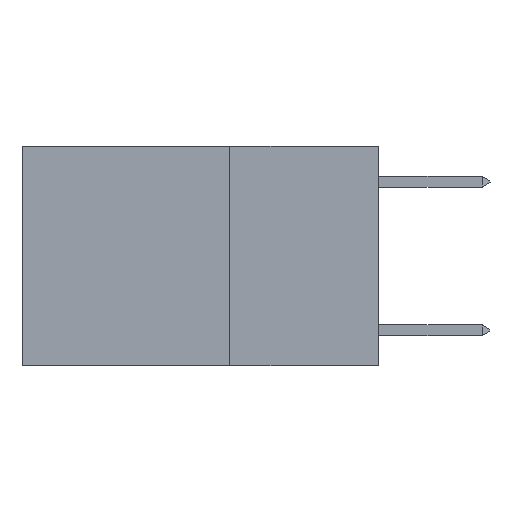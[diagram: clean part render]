
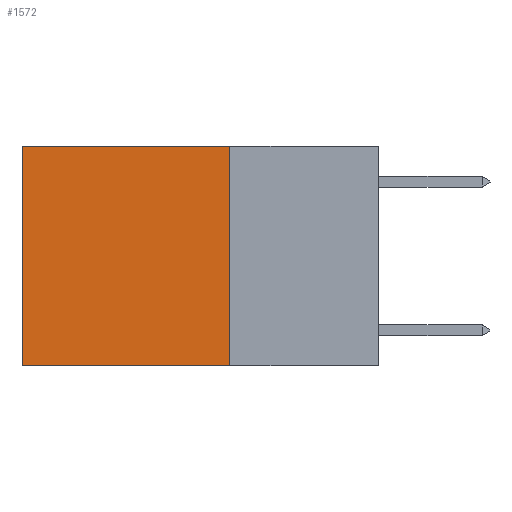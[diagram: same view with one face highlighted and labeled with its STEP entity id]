
A CAD part, left-side view. The second image highlights one B-rep face of the part: STEP entity #1572.
In plain terms, the highlighted planar face has unit normal (-1, 0, 0).
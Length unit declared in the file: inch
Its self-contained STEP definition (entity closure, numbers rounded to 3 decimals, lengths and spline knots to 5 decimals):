
#103 = VECTOR ( 'NONE', #2757, 39.37008 ) ;
#230 = CARTESIAN_POINT ( 'NONE',  ( 0.2625, 0.25, -0.37 ) ) ;
#568 = ORIENTED_EDGE ( 'NONE', *, *, #9293, .T. ) ;
#684 = ORIENTED_EDGE ( 'NONE', *, *, #6577, .F. ) ;
#697 = ORIENTED_EDGE ( 'NONE', *, *, #6767, .F. ) ;
#999 = DIRECTION ( 'NONE',  ( 0., 1., 0. ) ) ;
#1058 = ORIENTED_EDGE ( 'NONE', *, *, #4035, .T. ) ;
#1310 = CARTESIAN_POINT ( 'NONE',  ( 0.2625, 0.6, -0.37 ) ) ;
#1572 = ADVANCED_FACE ( 'NONE', ( #8146 ), #7570, .F. ) ;
#2045 = VECTOR ( 'NONE', #8404, 39.37008 ) ;
#2367 = LINE ( 'NONE', #3501, #2045 ) ;
#2757 = DIRECTION ( 'NONE',  ( 0., 1., 0. ) ) ;
#3449 = LINE ( 'NONE', #6725, #5382 ) ;
#3451 = DIRECTION ( 'NONE',  ( 0., 0., -1. ) ) ;
#3501 = CARTESIAN_POINT ( 'NONE',  ( 0.2625, 0.25, 0. ) ) ;
#3586 = VERTEX_POINT ( 'NONE', #7131 ) ;
#3865 = VERTEX_POINT ( 'NONE', #230 ) ;
#4035 = EDGE_CURVE ( 'NONE', #3586, #7804, #3449, .T. ) ;
#4064 = EDGE_LOOP ( 'NONE', ( #1058, #697, #684, #568 ) ) ;
#4070 = CARTESIAN_POINT ( 'NONE',  ( 0.2625, 0.25, 0. ) ) ;
#4244 = DIRECTION ( 'NONE',  ( 0., 0., -1. ) ) ;
#5070 = CARTESIAN_POINT ( 'NONE',  ( 0.2625, 0.25, 0. ) ) ;
#5382 = VECTOR ( 'NONE', #4244, 39.37008 ) ;
#6330 = VERTEX_POINT ( 'NONE', #4070 ) ;
#6349 = CARTESIAN_POINT ( 'NONE',  ( 0.2625, 0.25, 0. ) ) ;
#6577 = EDGE_CURVE ( 'NONE', #6330, #3865, #2367, .T. ) ;
#6725 = CARTESIAN_POINT ( 'NONE',  ( 0.2625, 0.6, 0. ) ) ;
#6767 = EDGE_CURVE ( 'NONE', #3865, #7804, #9174, .T. ) ;
#7131 = CARTESIAN_POINT ( 'NONE',  ( 0.2625, 0.6, 0. ) ) ;
#7570 = PLANE ( 'NONE',  #9556 ) ;
#7804 = VERTEX_POINT ( 'NONE', #1310 ) ;
#8146 = FACE_OUTER_BOUND ( 'NONE', #4064, .T. ) ;
#8358 = DIRECTION ( 'NONE',  ( 1., 0., 0. ) ) ;
#8404 = DIRECTION ( 'NONE',  ( 0., 0., -1. ) ) ;
#8541 = VECTOR ( 'NONE', #999, 39.37008 ) ;
#9174 = LINE ( 'NONE', #10981, #103 ) ;
#9293 = EDGE_CURVE ( 'NONE', #6330, #3586, #10758, .T. ) ;
#9556 = AXIS2_PLACEMENT_3D ( 'NONE', #5070, #8358, #3451 ) ;
#10758 = LINE ( 'NONE', #6349, #8541 ) ;
#10981 = CARTESIAN_POINT ( 'NONE',  ( 0.2625, 0.25, -0.37 ) ) ;
